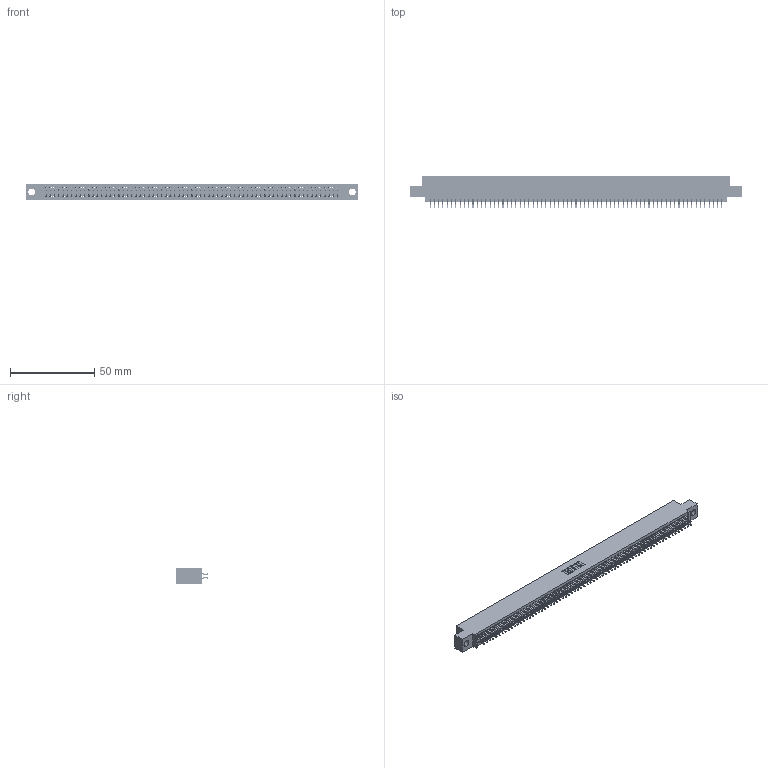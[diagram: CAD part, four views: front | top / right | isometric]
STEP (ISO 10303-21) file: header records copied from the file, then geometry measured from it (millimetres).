
FILE_DESCRIPTION (( 'STEP AP203' ), '1' );
FILE_NAME ('345-138-556-504.STEP', '2018-10-20T20:20:54', ( '' ), ( '' ), 'SwSTEP 2.0', 'SolidWorks 2016', '' );
FILE_SCHEMA (( 'CONFIG_CONTROL_DESIGN' ));
Length unit declared in the file: inch
Products named in the file (3): 345-138-556-504; 345-292-001_556 Tail; 345 Part_0.110 Offset - 0.156 Dia-TH
Assembly tree (139 placements, depth 2):
  345-138-556-504
    345 Part_0.110 Offset - 0.156 Dia-TH
    345-292-001_556 Tail  x138
Bounding box: 196.47 x 19.24 x 9.4 mm (x, y, z)
Volume: 19169.1 mm3; surface area: 28645.3 mm2
Topology: 139 solids, 139 shells, 7858 faces, 23399 edges, 15414 vertices
Faces by surface type: plane 5190, cylinder 2668
Entity records: 50859 total; most frequent: CARTESIAN_POINT 8516, ORIENTED_EDGE 8438, DIRECTION 7463, EDGE_CURVE 4219, VECTOR 3803, LINE 3803, VERTEX_POINT 2810, AXIS2_PLACEMENT_3D 1830
